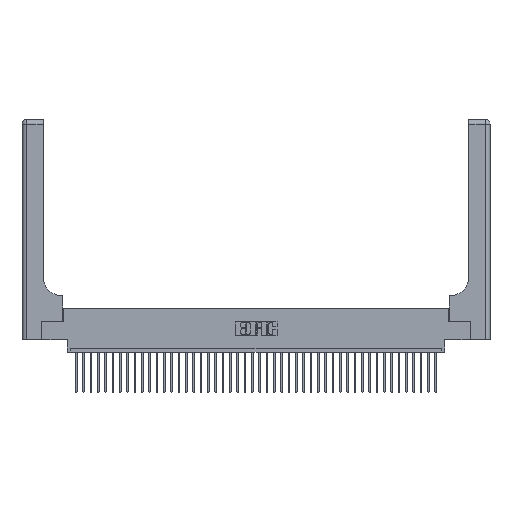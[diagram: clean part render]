
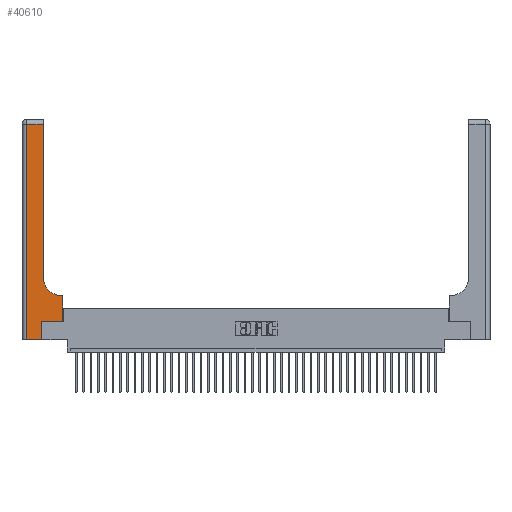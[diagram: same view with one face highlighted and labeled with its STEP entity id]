
A CAD part, top view. The second image highlights one B-rep face of the part: STEP entity #40610.
In plain terms, the highlighted planar face has unit normal (0, 0, 1).
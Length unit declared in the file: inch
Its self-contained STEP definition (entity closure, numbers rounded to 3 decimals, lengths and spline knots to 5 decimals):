
#2 = ORIENTED_EDGE ( 'NONE', *, *, #29945, .T. ) ;
#144 = VECTOR ( 'NONE', #39913, 39.37008 ) ;
#1125 = CARTESIAN_POINT ( 'NONE',  ( 0.269, 0., 0.37 ) ) ;
#1205 = DIRECTION ( 'NONE',  ( 0., 0., -1. ) ) ;
#1221 = ORIENTED_EDGE ( 'NONE', *, *, #40575, .T. ) ;
#1481 = EDGE_CURVE ( 'NONE', #14542, #40075, #19504, .T. ) ;
#1897 = VERTEX_POINT ( 'NONE', #5288 ) ;
#2260 = VECTOR ( 'NONE', #27948, 39.37008 ) ;
#2796 = LINE ( 'NONE', #11863, #11320 ) ;
#3127 = EDGE_CURVE ( 'NONE', #1897, #26023, #26905, .T. ) ;
#3577 = DIRECTION ( 'NONE',  ( 0., 0., -1. ) ) ;
#3894 = DIRECTION ( 'NONE',  ( 0., -1., 0. ) ) ;
#4442 = CARTESIAN_POINT ( 'NONE',  ( 0., 3., 0.37 ) ) ;
#4520 = VECTOR ( 'NONE', #9369, 39.37008 ) ;
#4915 = VERTEX_POINT ( 'NONE', #13027 ) ;
#5288 = CARTESIAN_POINT ( 'NONE',  ( 0.5585, 0.25, 0.37 ) ) ;
#6144 = EDGE_CURVE ( 'NONE', #4915, #20041, #14091, .T. ) ;
#6593 = EDGE_CURVE ( 'NONE', #26023, #14542, #33544, .T. ) ;
#7027 = LINE ( 'NONE', #41375, #4520 ) ;
#8131 = CARTESIAN_POINT ( 'NONE',  ( 0.5585, 0.6, 0.37 ) ) ;
#9369 = DIRECTION ( 'NONE',  ( 1., 0., 0. ) ) ;
#9646 = CARTESIAN_POINT ( 'NONE',  ( 0.06, 2.94, 0.37 ) ) ;
#10383 = VECTOR ( 'NONE', #37667, 39.37008 ) ;
#11320 = VECTOR ( 'NONE', #15519, 39.37008 ) ;
#11863 = CARTESIAN_POINT ( 'NONE',  ( 0., 0., 0.37 ) ) ;
#12129 = VECTOR ( 'NONE', #39088, 39.37008 ) ;
#13005 = DIRECTION ( 'NONE',  ( 0., 1., 0. ) ) ;
#13027 = CARTESIAN_POINT ( 'NONE',  ( 0.2915, 2.94, 0.37 ) ) ;
#13161 = CARTESIAN_POINT ( 'NONE',  ( 0.5415, 0.85, 0.37 ) ) ;
#14091 = LINE ( 'NONE', #35567, #12129 ) ;
#14542 = VERTEX_POINT ( 'NONE', #33112 ) ;
#15063 = ORIENTED_EDGE ( 'NONE', *, *, #6593, .T. ) ;
#15519 = DIRECTION ( 'NONE',  ( 1., 0., 0. ) ) ;
#15586 = VERTEX_POINT ( 'NONE', #1125 ) ;
#16774 = ORIENTED_EDGE ( 'NONE', *, *, #1481, .T. ) ;
#17824 = CARTESIAN_POINT ( 'NONE',  ( 0.269, 0.25, 0.37 ) ) ;
#18265 = EDGE_LOOP ( 'NONE', ( #1221, #22518, #36951, #31790, #2, #23375, #39045, #15063, #16774 ) ) ;
#19358 = VECTOR ( 'NONE', #13005, 39.37008 ) ;
#19504 = CIRCLE ( 'NONE', #25722, 0.25 ) ;
#20041 = VERTEX_POINT ( 'NONE', #9646 ) ;
#20303 = LINE ( 'NONE', #23479, #144 ) ;
#22518 = ORIENTED_EDGE ( 'NONE', *, *, #6144, .T. ) ;
#23375 = ORIENTED_EDGE ( 'NONE', *, *, #33344, .T. ) ;
#23479 = CARTESIAN_POINT ( 'NONE',  ( 0.2915, 3., 0.37 ) ) ;
#25343 = VERTEX_POINT ( 'NONE', #32257 ) ;
#25722 = AXIS2_PLACEMENT_3D ( 'NONE', #13161, #3577, #32638 ) ;
#26023 = VERTEX_POINT ( 'NONE', #8131 ) ;
#26905 = LINE ( 'NONE', #32098, #19358 ) ;
#27230 = CARTESIAN_POINT ( 'NONE',  ( 0.2915, 0.85, 0.37 ) ) ;
#27296 = CARTESIAN_POINT ( 'NONE',  ( 0.269, 0., 0.37 ) ) ;
#27948 = DIRECTION ( 'NONE',  ( -1., 0., 0. ) ) ;
#29945 = EDGE_CURVE ( 'NONE', #15586, #39583, #30099, .T. ) ;
#29995 = CARTESIAN_POINT ( 'NONE',  ( 0.06, 3., 0.37 ) ) ;
#30031 = VECTOR ( 'NONE', #3894, 39.37008 ) ;
#30099 = LINE ( 'NONE', #27296, #10383 ) ;
#30265 = DIRECTION ( 'NONE',  ( -1., 0., 0. ) ) ;
#31504 = EDGE_CURVE ( 'NONE', #25343, #15586, #2796, .T. ) ;
#31790 = ORIENTED_EDGE ( 'NONE', *, *, #31504, .T. ) ;
#32098 = CARTESIAN_POINT ( 'NONE',  ( 0.5585, 0.25, 0.37 ) ) ;
#32257 = CARTESIAN_POINT ( 'NONE',  ( 0.06, 0., 0.37 ) ) ;
#32638 = DIRECTION ( 'NONE',  ( 1., 0., 0. ) ) ;
#33112 = CARTESIAN_POINT ( 'NONE',  ( 0.5415, 0.6, 0.37 ) ) ;
#33344 = EDGE_CURVE ( 'NONE', #39583, #1897, #7027, .T. ) ;
#33544 = LINE ( 'NONE', #34424, #2260 ) ;
#34424 = CARTESIAN_POINT ( 'NONE',  ( 0.2915, 0.6, 0.37 ) ) ;
#35018 = FACE_OUTER_BOUND ( 'NONE', #18265, .T. ) ;
#35567 = CARTESIAN_POINT ( 'NONE',  ( 0., 2.94, 0.37 ) ) ;
#36323 = AXIS2_PLACEMENT_3D ( 'NONE', #4442, #1205, #30265 ) ;
#36377 = PLANE ( 'NONE',  #36323 ) ;
#36689 = EDGE_CURVE ( 'NONE', #20041, #25343, #38254, .T. ) ;
#36951 = ORIENTED_EDGE ( 'NONE', *, *, #36689, .T. ) ;
#37667 = DIRECTION ( 'NONE',  ( 0., 1., 0. ) ) ;
#38254 = LINE ( 'NONE', #29995, #30031 ) ;
#39045 = ORIENTED_EDGE ( 'NONE', *, *, #3127, .T. ) ;
#39088 = DIRECTION ( 'NONE',  ( -1., 0., 0. ) ) ;
#39583 = VERTEX_POINT ( 'NONE', #17824 ) ;
#39913 = DIRECTION ( 'NONE',  ( 0., 1., 0. ) ) ;
#40075 = VERTEX_POINT ( 'NONE', #27230 ) ;
#40575 = EDGE_CURVE ( 'NONE', #40075, #4915, #20303, .T. ) ;
#40610 = ADVANCED_FACE ( 'NONE', ( #35018 ), #36377, .F. ) ;
#41375 = CARTESIAN_POINT ( 'NONE',  ( 0.269, 0.25, 0.37 ) ) ;
